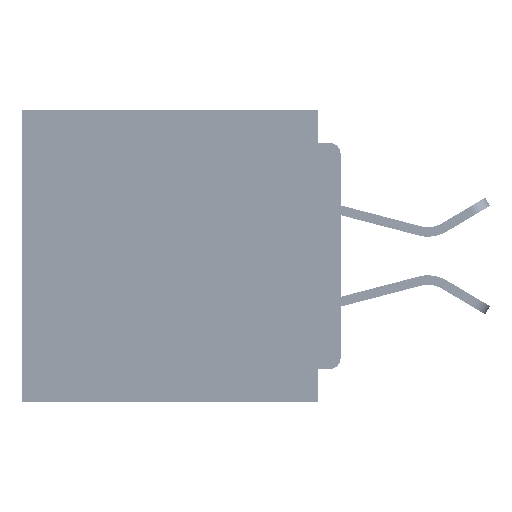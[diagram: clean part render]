
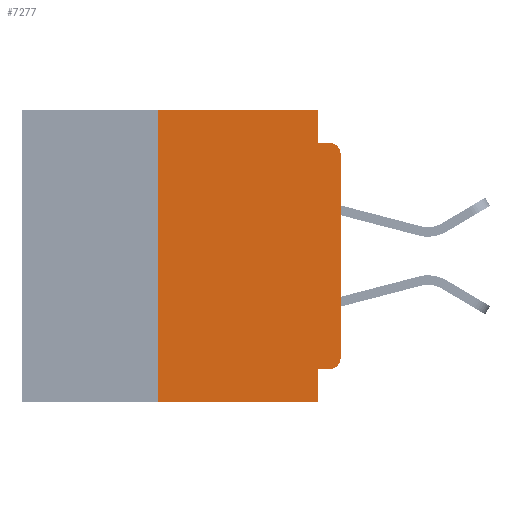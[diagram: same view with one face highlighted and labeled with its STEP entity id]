
A CAD part, left-side view. The second image highlights one B-rep face of the part: STEP entity #7277.
In plain terms, the highlighted planar face has unit normal (-1, 0, 0).
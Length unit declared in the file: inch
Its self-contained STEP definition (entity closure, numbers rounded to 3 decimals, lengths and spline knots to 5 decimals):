
#1715 = CARTESIAN_POINT ( 'NONE',  ( 0., 0.031, 0. ) ) ;
#4061 = AXIS2_PLACEMENT_3D ( 'NONE', #22778, #60413, #28252 ) ;
#5159 = LINE ( 'NONE', #45854, #62373 ) ;
#5915 = VECTOR ( 'NONE', #27200, 39.37008 ) ;
#6211 = CARTESIAN_POINT ( 'NONE',  ( 0., 0.437, 0. ) ) ;
#6260 = DIRECTION ( 'NONE',  ( 0., 0., 1. ) ) ;
#6774 = VECTOR ( 'NONE', #55550, 39.37008 ) ;
#7277 = ADVANCED_FACE ( 'NONE', ( #26502 ), #38489, .F. ) ;
#7762 = ORIENTED_EDGE ( 'NONE', *, *, #64991, .F. ) ;
#8165 = ORIENTED_EDGE ( 'NONE', *, *, #51311, .F. ) ;
#8744 = CARTESIAN_POINT ( 'NONE',  ( 0., 0., -0.355 ) ) ;
#9122 = ORIENTED_EDGE ( 'NONE', *, *, #55341, .T. ) ;
#10006 = CARTESIAN_POINT ( 'NONE',  ( 0., 0.031, 0. ) ) ;
#10246 = DIRECTION ( 'NONE',  ( 0., 0., -1. ) ) ;
#10848 = CARTESIAN_POINT ( 'NONE',  ( 0., 0., -0.34 ) ) ;
#11273 = DIRECTION ( 'NONE',  ( 0., -1., 0. ) ) ;
#11653 = DIRECTION ( 'NONE',  ( 1., 0., 0. ) ) ;
#12197 = LINE ( 'NONE', #10006, #67603 ) ;
#12511 = CARTESIAN_POINT ( 'NONE',  ( 0., 0.437, -0.4 ) ) ;
#13270 = CARTESIAN_POINT ( 'NONE',  ( 0., 0.015, -0.355 ) ) ;
#14400 = VERTEX_POINT ( 'NONE', #31351 ) ;
#18017 = VERTEX_POINT ( 'NONE', #35068 ) ;
#19407 = ORIENTED_EDGE ( 'NONE', *, *, #61097, .T. ) ;
#21738 = CARTESIAN_POINT ( 'NONE',  ( 0., 0.031, -0.4 ) ) ;
#22778 = CARTESIAN_POINT ( 'NONE',  ( 0., 0.015, -0.34 ) ) ;
#23561 = CARTESIAN_POINT ( 'NONE',  ( 0., 0.031, -0.4 ) ) ;
#25006 = VERTEX_POINT ( 'NONE', #58252 ) ;
#26502 = FACE_OUTER_BOUND ( 'NONE', #49854, .T. ) ;
#27200 = DIRECTION ( 'NONE',  ( 0., 0., -1. ) ) ;
#27571 = CARTESIAN_POINT ( 'NONE',  ( 0., 0.015, -0.06 ) ) ;
#27826 = LINE ( 'NONE', #65221, #54726 ) ;
#28252 = DIRECTION ( 'NONE',  ( 0., 0., -1. ) ) ;
#28578 = CARTESIAN_POINT ( 'NONE',  ( 0., 0.031, -0.045 ) ) ;
#28859 = VERTEX_POINT ( 'NONE', #13270 ) ;
#29343 = CARTESIAN_POINT ( 'NONE',  ( 0., 0., 0. ) ) ;
#31351 = CARTESIAN_POINT ( 'NONE',  ( 0., 0., -0.06 ) ) ;
#31521 = EDGE_CURVE ( 'NONE', #18017, #37215, #5159, .T. ) ;
#33008 = DIRECTION ( 'NONE',  ( 0., 0., -1. ) ) ;
#33841 = ORIENTED_EDGE ( 'NONE', *, *, #61696, .T. ) ;
#33871 = VECTOR ( 'NONE', #11273, 39.37008 ) ;
#34604 = LINE ( 'NONE', #21738, #5915 ) ;
#35068 = CARTESIAN_POINT ( 'NONE',  ( 0., 0.25, 0. ) ) ;
#37100 = CIRCLE ( 'NONE', #68522, 0.015 ) ;
#37215 = VERTEX_POINT ( 'NONE', #1715 ) ;
#38489 = PLANE ( 'NONE',  #67994 ) ;
#39721 = LINE ( 'NONE', #8744, #52325 ) ;
#40254 = VERTEX_POINT ( 'NONE', #64340 ) ;
#40342 = EDGE_CURVE ( 'NONE', #45082, #53621, #64028, .T. ) ;
#41012 = EDGE_CURVE ( 'NONE', #40254, #54995, #34604, .T. ) ;
#43297 = ORIENTED_EDGE ( 'NONE', *, *, #41012, .F. ) ;
#43484 = CARTESIAN_POINT ( 'NONE',  ( 0., 0., -0.045 ) ) ;
#45082 = VERTEX_POINT ( 'NONE', #28578 ) ;
#45178 = ORIENTED_EDGE ( 'NONE', *, *, #31521, .F. ) ;
#45638 = LINE ( 'NONE', #29343, #58228 ) ;
#45854 = CARTESIAN_POINT ( 'NONE',  ( 0., 0.437, 0. ) ) ;
#49276 = DIRECTION ( 'NONE',  ( 0., 0., -1. ) ) ;
#49610 = VERTEX_POINT ( 'NONE', #10848 ) ;
#49854 = EDGE_LOOP ( 'NONE', ( #54531, #9122, #60044, #7762, #45178, #55398, #19407, #43297, #8165, #33841 ) ) ;
#51270 = DIRECTION ( 'NONE',  ( 0., -1., 0. ) ) ;
#51311 = EDGE_CURVE ( 'NONE', #28859, #40254, #39721, .T. ) ;
#52325 = VECTOR ( 'NONE', #67862, 39.37008 ) ;
#52339 = EDGE_CURVE ( 'NONE', #25006, #18017, #27826, .T. ) ;
#53621 = VERTEX_POINT ( 'NONE', #65050 ) ;
#54531 = ORIENTED_EDGE ( 'NONE', *, *, #60117, .T. ) ;
#54726 = VECTOR ( 'NONE', #6260, 39.37008 ) ;
#54995 = VERTEX_POINT ( 'NONE', #23561 ) ;
#55341 = EDGE_CURVE ( 'NONE', #14400, #53621, #37100, .T. ) ;
#55398 = ORIENTED_EDGE ( 'NONE', *, *, #52339, .F. ) ;
#55494 = CIRCLE ( 'NONE', #4061, 0.015 ) ;
#55550 = DIRECTION ( 'NONE',  ( 0., -1., 0. ) ) ;
#58228 = VECTOR ( 'NONE', #66792, 39.37008 ) ;
#58252 = CARTESIAN_POINT ( 'NONE',  ( 0., 0.25, -0.4 ) ) ;
#60044 = ORIENTED_EDGE ( 'NONE', *, *, #40342, .F. ) ;
#60117 = EDGE_CURVE ( 'NONE', #49610, #14400, #45638, .T. ) ;
#60413 = DIRECTION ( 'NONE',  ( -1., 0., 0. ) ) ;
#61097 = EDGE_CURVE ( 'NONE', #25006, #54995, #63916, .T. ) ;
#61696 = EDGE_CURVE ( 'NONE', #28859, #49610, #55494, .T. ) ;
#62373 = VECTOR ( 'NONE', #51270, 39.37008 ) ;
#63916 = LINE ( 'NONE', #12511, #6774 ) ;
#64028 = LINE ( 'NONE', #43484, #33871 ) ;
#64340 = CARTESIAN_POINT ( 'NONE',  ( 0., 0.031, -0.355 ) ) ;
#64991 = EDGE_CURVE ( 'NONE', #37215, #45082, #12197, .T. ) ;
#65050 = CARTESIAN_POINT ( 'NONE',  ( 0., 0.015, -0.045 ) ) ;
#65060 = DIRECTION ( 'NONE',  ( -1., 0., 0. ) ) ;
#65221 = CARTESIAN_POINT ( 'NONE',  ( 0., 0.25, -0.4 ) ) ;
#66792 = DIRECTION ( 'NONE',  ( 0., 0., 1. ) ) ;
#67603 = VECTOR ( 'NONE', #10246, 39.37008 ) ;
#67862 = DIRECTION ( 'NONE',  ( 0., 1., 0. ) ) ;
#67994 = AXIS2_PLACEMENT_3D ( 'NONE', #6211, #11653, #49276 ) ;
#68522 = AXIS2_PLACEMENT_3D ( 'NONE', #27571, #65060, #33008 ) ;
